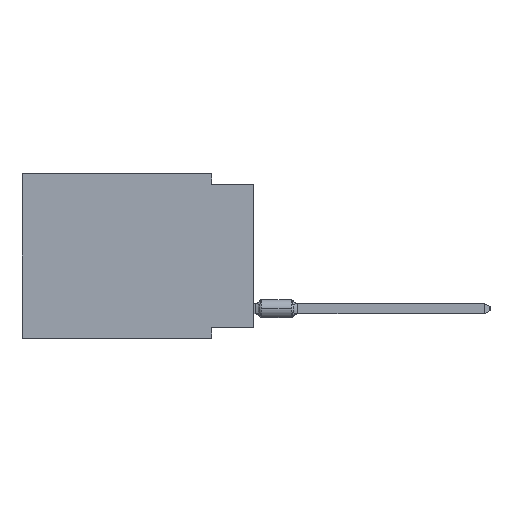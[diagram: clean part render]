
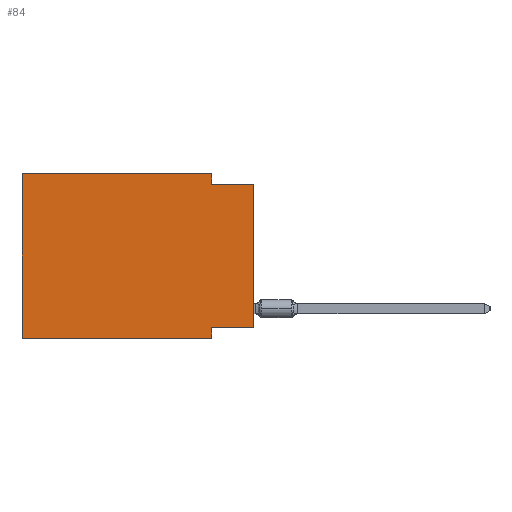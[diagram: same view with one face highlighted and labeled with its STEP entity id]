
A CAD part, left-side view. The second image highlights one B-rep face of the part: STEP entity #84.
In plain terms, the highlighted planar face has unit normal (-1, 0, 0).
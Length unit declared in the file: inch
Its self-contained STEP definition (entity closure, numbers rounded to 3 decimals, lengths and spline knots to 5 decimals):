
#84 = ADVANCED_FACE ( 'NONE', ( #31535 ), #84221, .F. ) ;
#987 = EDGE_CURVE ( 'NONE', #71928, #32048, #71925, .T. ) ;
#1008 = AXIS2_PLACEMENT_3D ( 'NONE', #23795, #3968, #16479 ) ;
#1459 = CARTESIAN_POINT ( 'NONE',  ( 0., 0., -0.365 ) ) ;
#2838 = EDGE_CURVE ( 'NONE', #41496, #71928, #70443, .T. ) ;
#2918 = VECTOR ( 'NONE', #37906, 39.37008 ) ;
#3858 = CARTESIAN_POINT ( 'NONE',  ( 0., 0., -0.025 ) ) ;
#3968 = DIRECTION ( 'NONE',  ( 1., 0., 0. ) ) ;
#4324 = CARTESIAN_POINT ( 'NONE',  ( 0., 0.1, -0.39 ) ) ;
#5598 = DIRECTION ( 'NONE',  ( 0., 0., -1. ) ) ;
#5914 = VERTEX_POINT ( 'NONE', #21143 ) ;
#6045 = EDGE_CURVE ( 'NONE', #81991, #68668, #69484, .T. ) ;
#7298 = CARTESIAN_POINT ( 'NONE',  ( 0., 0.1, -0.025 ) ) ;
#7610 = LINE ( 'NONE', #20119, #44324 ) ;
#11588 = LINE ( 'NONE', #38749, #84922 ) ;
#11646 = CARTESIAN_POINT ( 'NONE',  ( 0., 0.1, 0. ) ) ;
#15193 = ORIENTED_EDGE ( 'NONE', *, *, #6045, .F. ) ;
#16479 = DIRECTION ( 'NONE',  ( 0., 0., -1. ) ) ;
#18170 = CARTESIAN_POINT ( 'NONE',  ( 0., 0., -0.365 ) ) ;
#19690 = ORIENTED_EDGE ( 'NONE', *, *, #24460, .F. ) ;
#20119 = CARTESIAN_POINT ( 'NONE',  ( 0., 0.55, -0.39 ) ) ;
#21143 = CARTESIAN_POINT ( 'NONE',  ( 0., 0.55, 0. ) ) ;
#21757 = VERTEX_POINT ( 'NONE', #34704 ) ;
#23795 = CARTESIAN_POINT ( 'NONE',  ( 0., 0.55, 0. ) ) ;
#24460 = EDGE_CURVE ( 'NONE', #21757, #81991, #38806, .T. ) ;
#26995 = DIRECTION ( 'NONE',  ( 0., 0., -1. ) ) ;
#28299 = DIRECTION ( 'NONE',  ( 0., -1., 0. ) ) ;
#28355 = CARTESIAN_POINT ( 'NONE',  ( 0., 0.55, 0. ) ) ;
#29259 = ORIENTED_EDGE ( 'NONE', *, *, #51891, .T. ) ;
#31535 = FACE_OUTER_BOUND ( 'NONE', #49852, .T. ) ;
#32048 = VERTEX_POINT ( 'NONE', #4324 ) ;
#34704 = CARTESIAN_POINT ( 'NONE',  ( 0., 0.1, 0. ) ) ;
#34961 = VECTOR ( 'NONE', #56183, 39.37008 ) ;
#35049 = EDGE_CURVE ( 'NONE', #5914, #21757, #52979, .T. ) ;
#35466 = ORIENTED_EDGE ( 'NONE', *, *, #987, .F. ) ;
#35780 = VERTEX_POINT ( 'NONE', #48162 ) ;
#36433 = CARTESIAN_POINT ( 'NONE',  ( 0., 0.1, -0.365 ) ) ;
#37906 = DIRECTION ( 'NONE',  ( 0., -1., 0. ) ) ;
#38588 = ORIENTED_EDGE ( 'NONE', *, *, #71299, .F. ) ;
#38749 = CARTESIAN_POINT ( 'NONE',  ( 0., 0.55, 0. ) ) ;
#38806 = LINE ( 'NONE', #11646, #81246 ) ;
#40454 = VECTOR ( 'NONE', #26995, 39.37008 ) ;
#41496 = VERTEX_POINT ( 'NONE', #1459 ) ;
#44324 = VECTOR ( 'NONE', #28299, 39.37008 ) ;
#48064 = DIRECTION ( 'NONE',  ( 0., 0., 1. ) ) ;
#48162 = CARTESIAN_POINT ( 'NONE',  ( 0., 0.55, -0.39 ) ) ;
#49852 = EDGE_LOOP ( 'NONE', ( #72295, #15193, #19690, #77536, #38588, #29259, #35466, #63835 ) ) ;
#51891 = EDGE_CURVE ( 'NONE', #35780, #32048, #7610, .T. ) ;
#52979 = LINE ( 'NONE', #28355, #58646 ) ;
#53394 = EDGE_CURVE ( 'NONE', #41496, #68668, #67514, .T. ) ;
#53692 = CARTESIAN_POINT ( 'NONE',  ( 0., 0., 0. ) ) ;
#56183 = DIRECTION ( 'NONE',  ( 0., 1., 0. ) ) ;
#58646 = VECTOR ( 'NONE', #67653, 39.37008 ) ;
#63835 = ORIENTED_EDGE ( 'NONE', *, *, #2838, .F. ) ;
#65445 = CARTESIAN_POINT ( 'NONE',  ( 0., 0.1, -0.39 ) ) ;
#67514 = LINE ( 'NONE', #53692, #83164 ) ;
#67653 = DIRECTION ( 'NONE',  ( 0., -1., 0. ) ) ;
#68668 = VERTEX_POINT ( 'NONE', #81376 ) ;
#69484 = LINE ( 'NONE', #3858, #2918 ) ;
#70443 = LINE ( 'NONE', #18170, #34961 ) ;
#71299 = EDGE_CURVE ( 'NONE', #35780, #5914, #11588, .T. ) ;
#71925 = LINE ( 'NONE', #65445, #40454 ) ;
#71928 = VERTEX_POINT ( 'NONE', #36433 ) ;
#72295 = ORIENTED_EDGE ( 'NONE', *, *, #53394, .T. ) ;
#77536 = ORIENTED_EDGE ( 'NONE', *, *, #35049, .F. ) ;
#78082 = DIRECTION ( 'NONE',  ( 0., 0., 1. ) ) ;
#81246 = VECTOR ( 'NONE', #5598, 39.37008 ) ;
#81376 = CARTESIAN_POINT ( 'NONE',  ( 0., 0., -0.025 ) ) ;
#81991 = VERTEX_POINT ( 'NONE', #7298 ) ;
#83164 = VECTOR ( 'NONE', #48064, 39.37008 ) ;
#84221 = PLANE ( 'NONE',  #1008 ) ;
#84922 = VECTOR ( 'NONE', #78082, 39.37008 ) ;
